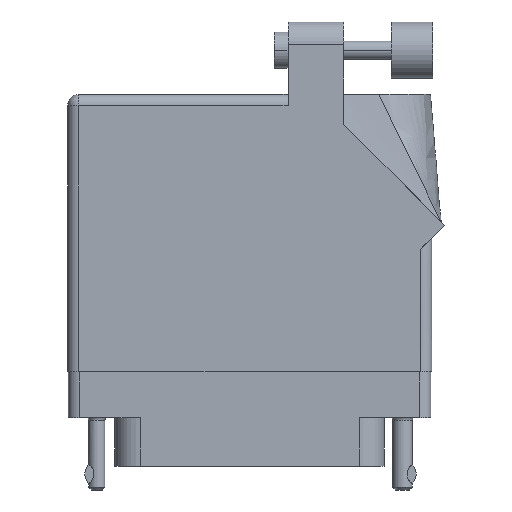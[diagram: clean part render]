
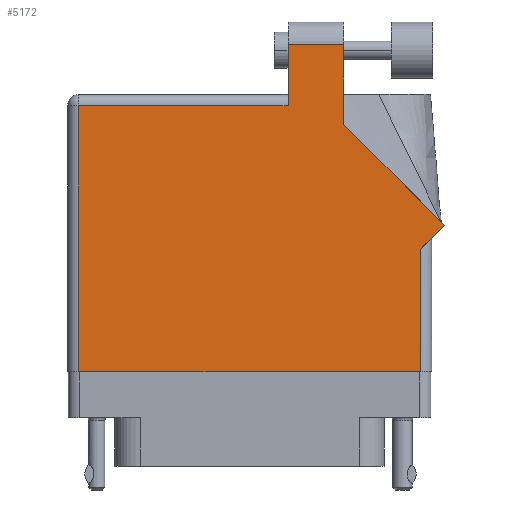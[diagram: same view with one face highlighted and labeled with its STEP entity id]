
A CAD part, front view. The second image highlights one B-rep face of the part: STEP entity #5172.
In plain terms, the highlighted face is planar.
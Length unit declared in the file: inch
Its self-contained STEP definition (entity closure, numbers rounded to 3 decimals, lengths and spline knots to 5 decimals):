
#206 = CARTESIAN_POINT ( 'NONE',  ( 0.212, 1.705, 0.455 ) ) ;
#1220 = VECTOR ( 'NONE', #1256, 39.37008 ) ;
#1256 = DIRECTION ( 'NONE',  ( -0.707, 0.707, 0. ) ) ;
#1683 = CARTESIAN_POINT ( 'NONE',  ( 0.943, 0.575, 0.455 ) ) ;
#1954 = DIRECTION ( 'NONE',  ( -1., 0., 0. ) ) ;
#2172 = DIRECTION ( 'NONE',  ( -1., 0., 0. ) ) ;
#2810 = CARTESIAN_POINT ( 'NONE',  ( 0.212, 1.43, 0.455 ) ) ;
#4464 = VERTEX_POINT ( 'NONE', #12404 ) ;
#4651 = ORIENTED_EDGE ( 'NONE', *, *, #39620, .T. ) ;
#4817 = CARTESIAN_POINT ( 'NONE',  ( 0.519, 1.26442, 0.455 ) ) ;
#5172 = ADVANCED_FACE ( 'NONE', ( #40241 ), #27841, .F. ) ;
#5740 = EDGE_CURVE ( 'NONE', #35360, #6219, #29290, .T. ) ;
#5804 = CARTESIAN_POINT ( 'NONE',  ( -1.005, -0.1, 0.455 ) ) ;
#5958 = DIRECTION ( 'NONE',  ( -1., 0., 0. ) ) ;
#6219 = VERTEX_POINT ( 'NONE', #34642 ) ;
#7901 = CARTESIAN_POINT ( 'NONE',  ( -0.943, 1.368, 0.455 ) ) ;
#8871 = LINE ( 'NONE', #39336, #16599 ) ;
#8916 = CARTESIAN_POINT ( 'NONE',  ( -1.005, 1.43, 0.455 ) ) ;
#9397 = CARTESIAN_POINT ( 'NONE',  ( 1.07571, 0.70771, 0.455 ) ) ;
#10928 = EDGE_LOOP ( 'NONE', ( #18574, #48351, #18877, #12335, #13305, #4651, #12848, #46861, #22568 ) ) ;
#11089 = CARTESIAN_POINT ( 'NONE',  ( -0.943, -0.1, 0.455 ) ) ;
#11222 = DIRECTION ( 'NONE',  ( 1., 0., 0. ) ) ;
#11904 = LINE ( 'NONE', #9397, #1220 ) ;
#12335 = ORIENTED_EDGE ( 'NONE', *, *, #36611, .T. ) ;
#12404 = CARTESIAN_POINT ( 'NONE',  ( -0.943, -0.1, 0.455 ) ) ;
#12848 = ORIENTED_EDGE ( 'NONE', *, *, #23596, .T. ) ;
#13051 = LINE ( 'NONE', #22727, #27900 ) ;
#13064 = VERTEX_POINT ( 'NONE', #7901 ) ;
#13240 = DIRECTION ( 'NONE',  ( 0., 0., -1. ) ) ;
#13305 = ORIENTED_EDGE ( 'NONE', *, *, #46732, .T. ) ;
#15922 = VECTOR ( 'NONE', #19908, 39.37008 ) ;
#16077 = VERTEX_POINT ( 'NONE', #16277 ) ;
#16277 = CARTESIAN_POINT ( 'NONE',  ( 0.943, -0.1, 0.455 ) ) ;
#16599 = VECTOR ( 'NONE', #2172, 39.37008 ) ;
#18574 = ORIENTED_EDGE ( 'NONE', *, *, #24903, .T. ) ;
#18741 = DIRECTION ( 'NONE',  ( 0., -1., 0. ) ) ;
#18877 = ORIENTED_EDGE ( 'NONE', *, *, #5740, .T. ) ;
#19824 = EDGE_CURVE ( 'NONE', #49178, #28563, #11904, .T. ) ;
#19908 = DIRECTION ( 'NONE',  ( 0., 1., 0. ) ) ;
#22568 = ORIENTED_EDGE ( 'NONE', *, *, #19824, .T. ) ;
#22727 = CARTESIAN_POINT ( 'NONE',  ( 0.943, 0.637, 0.455 ) ) ;
#23596 = EDGE_CURVE ( 'NONE', #16077, #32697, #13051, .T. ) ;
#24208 = DIRECTION ( 'NONE',  ( 0.707, 0.707, 0. ) ) ;
#24258 = CARTESIAN_POINT ( 'NONE',  ( 1.07571, 0.70771, 0.455 ) ) ;
#24753 = LINE ( 'NONE', #11089, #27702 ) ;
#24903 = EDGE_CURVE ( 'NONE', #28563, #28338, #32571, .T. ) ;
#25236 = VECTOR ( 'NONE', #24208, 39.37008 ) ;
#27702 = VECTOR ( 'NONE', #18741, 39.37008 ) ;
#27841 = PLANE ( 'NONE',  #44143 ) ;
#27900 = VECTOR ( 'NONE', #29885, 39.37008 ) ;
#28338 = VERTEX_POINT ( 'NONE', #32057 ) ;
#28563 = VERTEX_POINT ( 'NONE', #39986 ) ;
#29290 = LINE ( 'NONE', #2810, #31058 ) ;
#29885 = DIRECTION ( 'NONE',  ( 0., 1., 0. ) ) ;
#31058 = VECTOR ( 'NONE', #44135, 39.37008 ) ;
#31689 = CARTESIAN_POINT ( 'NONE',  ( 1.005, 0.637, 0.455 ) ) ;
#32057 = CARTESIAN_POINT ( 'NONE',  ( 0.519, 1.705, 0.455 ) ) ;
#32233 = EDGE_CURVE ( 'NONE', #32697, #49178, #48427, .T. ) ;
#32521 = CARTESIAN_POINT ( 'NONE',  ( 0.212, 1.705, 0.455 ) ) ;
#32571 = LINE ( 'NONE', #4817, #15922 ) ;
#32697 = VERTEX_POINT ( 'NONE', #1683 ) ;
#33465 = EDGE_CURVE ( 'NONE', #28338, #35360, #41769, .T. ) ;
#34642 = CARTESIAN_POINT ( 'NONE',  ( 0.212, 1.368, 0.455 ) ) ;
#35147 = VECTOR ( 'NONE', #11222, 39.37008 ) ;
#35360 = VERTEX_POINT ( 'NONE', #206 ) ;
#36611 = EDGE_CURVE ( 'NONE', #6219, #13064, #8871, .T. ) ;
#39336 = CARTESIAN_POINT ( 'NONE',  ( -1.005, 1.368, 0.455 ) ) ;
#39620 = EDGE_CURVE ( 'NONE', #4464, #16077, #40477, .T. ) ;
#39986 = CARTESIAN_POINT ( 'NONE',  ( 0.519, 1.26442, 0.455 ) ) ;
#40241 = FACE_OUTER_BOUND ( 'NONE', #10928, .T. ) ;
#40477 = LINE ( 'NONE', #5804, #35147 ) ;
#41769 = LINE ( 'NONE', #32521, #48910 ) ;
#44135 = DIRECTION ( 'NONE',  ( 0., -1., 0. ) ) ;
#44143 = AXIS2_PLACEMENT_3D ( 'NONE', #8916, #13240, #1954 ) ;
#46732 = EDGE_CURVE ( 'NONE', #13064, #4464, #24753, .T. ) ;
#46861 = ORIENTED_EDGE ( 'NONE', *, *, #32233, .T. ) ;
#48351 = ORIENTED_EDGE ( 'NONE', *, *, #33465, .T. ) ;
#48427 = LINE ( 'NONE', #31689, #25236 ) ;
#48910 = VECTOR ( 'NONE', #5958, 39.37008 ) ;
#49178 = VERTEX_POINT ( 'NONE', #24258 ) ;
